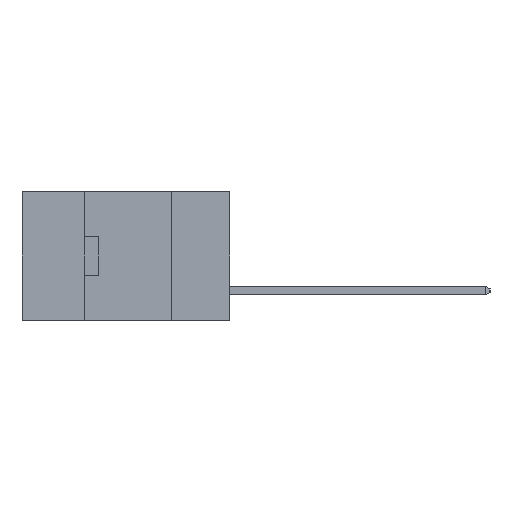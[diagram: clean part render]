
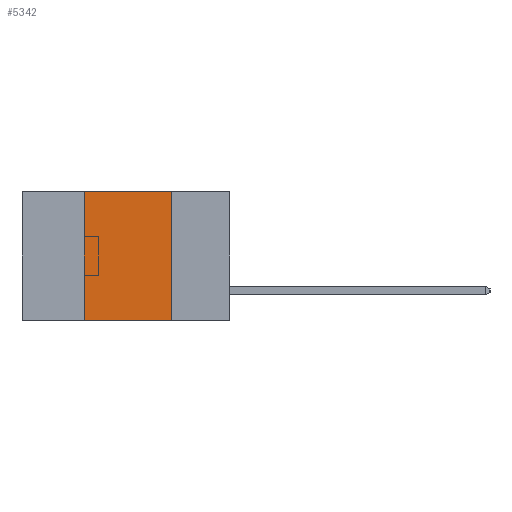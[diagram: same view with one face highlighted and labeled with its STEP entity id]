
A CAD part, left-side view. The second image highlights one B-rep face of the part: STEP entity #5342.
In plain terms, the highlighted planar face has unit normal (-1, 0, 0).
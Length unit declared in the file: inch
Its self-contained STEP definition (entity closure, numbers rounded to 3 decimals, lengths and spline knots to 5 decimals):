
#210 = VECTOR ( 'NONE', #11741, 39.37008 ) ;
#2086 = CARTESIAN_POINT ( 'NONE',  ( 0., 0.17, -0.37 ) ) ;
#2436 = ORIENTED_EDGE ( 'NONE', *, *, #24790, .F. ) ;
#2988 = EDGE_CURVE ( 'NONE', #4501, #5459, #22119, .T. ) ;
#4113 = CARTESIAN_POINT ( 'NONE',  ( 0., 0.17, 0. ) ) ;
#4501 = VERTEX_POINT ( 'NONE', #4534 ) ;
#4534 = CARTESIAN_POINT ( 'NONE',  ( 0., 0.42, 0. ) ) ;
#5342 = ADVANCED_FACE ( 'NONE', ( #7136 ), #10693, .F. ) ;
#5459 = VERTEX_POINT ( 'NONE', #4113 ) ;
#7136 = FACE_OUTER_BOUND ( 'NONE', #26699, .T. ) ;
#7342 = EDGE_CURVE ( 'NONE', #5459, #9139, #16730, .T. ) ;
#7515 = ORIENTED_EDGE ( 'NONE', *, *, #2988, .F. ) ;
#8380 = CARTESIAN_POINT ( 'NONE',  ( 0., 0.42, -0.37 ) ) ;
#9139 = VERTEX_POINT ( 'NONE', #2086 ) ;
#10425 = DIRECTION ( 'NONE',  ( 0., 0., -1. ) ) ;
#10568 = DIRECTION ( 'NONE',  ( 1., 0., 0. ) ) ;
#10656 = CARTESIAN_POINT ( 'NONE',  ( 0., 0.6, -0.37 ) ) ;
#10693 = PLANE ( 'NONE',  #17848 ) ;
#10846 = LINE ( 'NONE', #22760, #15189 ) ;
#11349 = CARTESIAN_POINT ( 'NONE',  ( 0., 0.6, 0. ) ) ;
#11689 = CARTESIAN_POINT ( 'NONE',  ( 0., 0.17, -0.37 ) ) ;
#11741 = DIRECTION ( 'NONE',  ( 0., 0., -1. ) ) ;
#13590 = DIRECTION ( 'NONE',  ( 0., -1., 0. ) ) ;
#13912 = ORIENTED_EDGE ( 'NONE', *, *, #17908, .T. ) ;
#14069 = CARTESIAN_POINT ( 'NONE',  ( 0., 0.6, 0. ) ) ;
#14285 = LINE ( 'NONE', #10656, #18575 ) ;
#15189 = VECTOR ( 'NONE', #26916, 39.37008 ) ;
#16583 = VECTOR ( 'NONE', #13590, 39.37008 ) ;
#16730 = LINE ( 'NONE', #11689, #210 ) ;
#17101 = DIRECTION ( 'NONE',  ( 0., -1., 0. ) ) ;
#17848 = AXIS2_PLACEMENT_3D ( 'NONE', #11349, #10568, #10425 ) ;
#17908 = EDGE_CURVE ( 'NONE', #19835, #9139, #14285, .T. ) ;
#18575 = VECTOR ( 'NONE', #17101, 39.37008 ) ;
#19835 = VERTEX_POINT ( 'NONE', #8380 ) ;
#22119 = LINE ( 'NONE', #14069, #16583 ) ;
#22760 = CARTESIAN_POINT ( 'NONE',  ( 0., 0.42, -0.37 ) ) ;
#23678 = ORIENTED_EDGE ( 'NONE', *, *, #7342, .F. ) ;
#24790 = EDGE_CURVE ( 'NONE', #19835, #4501, #10846, .T. ) ;
#26699 = EDGE_LOOP ( 'NONE', ( #23678, #7515, #2436, #13912 ) ) ;
#26916 = DIRECTION ( 'NONE',  ( 0., 0., 1. ) ) ;
